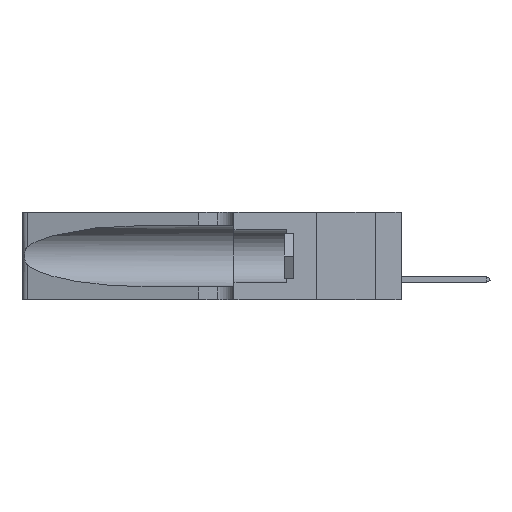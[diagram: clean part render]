
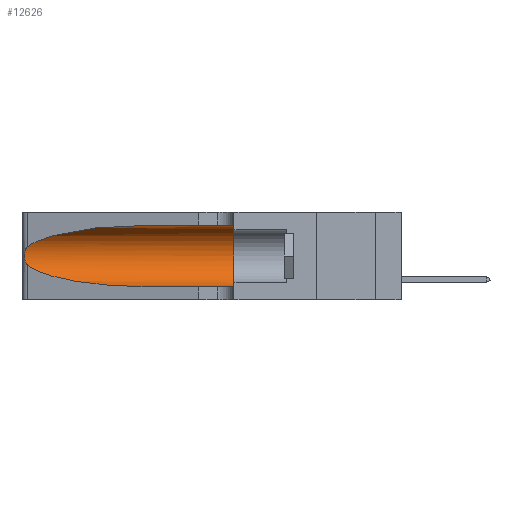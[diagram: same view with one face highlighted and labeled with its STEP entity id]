
A CAD part, left-side view. The second image highlights one B-rep face of the part: STEP entity #12626.
In plain terms, the highlighted cylindrical face has radius 3.308 mm (diameter 6.617 mm), a partial arc.
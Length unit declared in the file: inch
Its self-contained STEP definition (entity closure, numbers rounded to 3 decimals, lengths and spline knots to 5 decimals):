
#149 = DIRECTION ( 'NONE',  ( 0., 1., 0. ) ) ;
#244 = AXIS2_PLACEMENT_3D ( 'NONE', #2446, #10151, #14197 ) ;
#538 = CARTESIAN_POINT ( 'NONE',  ( 0.1305, 0.35, 0.05475 ) ) ;
#945 = CARTESIAN_POINT ( 'NONE',  ( 0.25487, 1.22718, 0.22369 ) ) ;
#1128 = EDGE_CURVE ( 'NONE', #13050, #4423, #2606, .T. ) ;
#2004 = ORIENTED_EDGE ( 'NONE', *, *, #10098, .T. ) ;
#2446 = CARTESIAN_POINT ( 'NONE',  ( 0.1305, 1.61858, 0.185 ) ) ;
#2606 = B_SPLINE_CURVE_WITH_KNOTS ( 'NONE', 3,
 ( #945, #4866, #18875, #8813, #20917, #10826, #5034, #8907, #22901, #22994, #10918, #24805, #25061, #9157 ),
 .UNSPECIFIED., .F., .F.,
 ( 4, 2, 2, 2, 2, 2, 4 ),
 ( 0., 0.00027, 0.00053, 0.00107, 0.0016, 0.00187, 0.00214 ),
 .UNSPECIFIED. ) ;
#3045 = FACE_OUTER_BOUND ( 'NONE', #23670, .T. ) ;
#3299 = DIRECTION ( 'NONE',  ( 0., -1., 0. ) ) ;
#4108 = CIRCLE ( 'NONE', #12021, 0.13025 ) ;
#4423 = VERTEX_POINT ( 'NONE', #16565 ) ;
#4842 = LINE ( 'NONE', #13563, #21802 ) ;
#4866 = CARTESIAN_POINT ( 'NONE',  ( 0.25555, 1.22994, 0.2215 ) ) ;
#5034 = CARTESIAN_POINT ( 'NONE',  ( 0.26075, 1.23896, 0.19203 ) ) ;
#5243 = CARTESIAN_POINT ( 'NONE',  ( 0.2373, 1.15595, 0.28018 ) ) ;
#6043 = VERTEX_POINT ( 'NONE', #14174 ) ;
#7356 = CARTESIAN_POINT ( 'NONE',  ( 0.18966, 0.96281, 0.31525 ) ) ;
#8057 =( BOUNDED_CURVE ( )  B_SPLINE_CURVE ( 3, ( #17282, #7356, #5243, #21306 ),
 .UNSPECIFIED., .F., .T. ) 
 B_SPLINE_CURVE_WITH_KNOTS ( ( 4, 4 ),
 ( 1.5708, 2.84003 ),
 .UNSPECIFIED. ) 
 CURVE ( )  GEOMETRIC_REPRESENTATION_ITEM ( )  RATIONAL_B_SPLINE_CURVE ( ( 1., 0.87, 0.87, 1. ) ) 
 REPRESENTATION_ITEM ( '' )  );
#8094 = VERTEX_POINT ( 'NONE', #538 ) ;
#8813 = CARTESIAN_POINT ( 'NONE',  ( 0.25787, 1.23484, 0.2124 ) ) ;
#8861 = CARTESIAN_POINT ( 'NONE',  ( 0.25487, 1.22718, 0.14631 ) ) ;
#8907 = CARTESIAN_POINT ( 'NONE',  ( 0.26075, 1.23896, 0.178 ) ) ;
#8988 = DIRECTION ( 'NONE',  ( 0., -1., 0. ) ) ;
#9157 = CARTESIAN_POINT ( 'NONE',  ( 0.25487, 1.22718, 0.14631 ) ) ;
#10098 = EDGE_CURVE ( 'NONE', #13844, #8094, #10925, .T. ) ;
#10126 = DIRECTION ( 'NONE',  ( 0., 0., 1. ) ) ;
#10151 = DIRECTION ( 'NONE',  ( 0., -1., 0. ) ) ;
#10527 = CARTESIAN_POINT ( 'NONE',  ( 0.2373, 1.15595, 0.08982 ) ) ;
#10826 = CARTESIAN_POINT ( 'NONE',  ( 0.26018, 1.23835, 0.19895 ) ) ;
#10918 = CARTESIAN_POINT ( 'NONE',  ( 0.25789, 1.23486, 0.15765 ) ) ;
#10925 = LINE ( 'NONE', #23768, #11554 ) ;
#11221 = CARTESIAN_POINT ( 'NONE',  ( 0.18966, 0.96281, 0.05475 ) ) ;
#11554 = VECTOR ( 'NONE', #8988, 39.37008 ) ;
#12021 = AXIS2_PLACEMENT_3D ( 'NONE', #12308, #149, #10126 ) ;
#12260 = CARTESIAN_POINT ( 'NONE',  ( 0.1305, 0.72297, 0.05475 ) ) ;
#12274 = CARTESIAN_POINT ( 'NONE',  ( 0.1305, 0.35, 0.31525 ) ) ;
#12308 = CARTESIAN_POINT ( 'NONE',  ( 0.1305, 0.35, 0.185 ) ) ;
#12352 = VERTEX_POINT ( 'NONE', #12274 ) ;
#12369 = EDGE_CURVE ( 'NONE', #4423, #13844, #13871, .T. ) ;
#12626 = ADVANCED_FACE ( 'NONE', ( #3045 ), #23665, .F. ) ;
#13050 = VERTEX_POINT ( 'NONE', #25778 ) ;
#13269 = CARTESIAN_POINT ( 'NONE',  ( 0.1305, 0.72297, 0.05475 ) ) ;
#13563 = CARTESIAN_POINT ( 'NONE',  ( 0.1305, 1.61858, 0.31525 ) ) ;
#13749 = ORIENTED_EDGE ( 'NONE', *, *, #1128, .T. ) ;
#13844 = VERTEX_POINT ( 'NONE', #12260 ) ;
#13871 =( BOUNDED_CURVE ( )  B_SPLINE_CURVE ( 3, ( #8861, #10527, #11221, #13269 ),
 .UNSPECIFIED., .F., .T. ) 
 B_SPLINE_CURVE_WITH_KNOTS ( ( 4, 4 ),
 ( 3.44316, 4.71239 ),
 .UNSPECIFIED. ) 
 CURVE ( )  GEOMETRIC_REPRESENTATION_ITEM ( )  RATIONAL_B_SPLINE_CURVE ( ( 1., 0.87, 0.87, 1. ) ) 
 REPRESENTATION_ITEM ( '' )  );
#14174 = CARTESIAN_POINT ( 'NONE',  ( 0.1305, 0.72297, 0.31525 ) ) ;
#14197 = DIRECTION ( 'NONE',  ( 0., 0., -1. ) ) ;
#14296 = ORIENTED_EDGE ( 'NONE', *, *, #15619, .F. ) ;
#15619 = EDGE_CURVE ( 'NONE', #12352, #8094, #4108, .T. ) ;
#16565 = CARTESIAN_POINT ( 'NONE',  ( 0.25487, 1.22718, 0.14631 ) ) ;
#16695 = ORIENTED_EDGE ( 'NONE', *, *, #21249, .F. ) ;
#17282 = CARTESIAN_POINT ( 'NONE',  ( 0.1305, 0.72297, 0.31525 ) ) ;
#18875 = CARTESIAN_POINT ( 'NONE',  ( 0.25639, 1.23184, 0.21858 ) ) ;
#18878 = ORIENTED_EDGE ( 'NONE', *, *, #12369, .T. ) ;
#20072 = EDGE_CURVE ( 'NONE', #6043, #13050, #8057, .T. ) ;
#20917 = CARTESIAN_POINT ( 'NONE',  ( 0.25854, 1.2359, 0.20912 ) ) ;
#21065 = ORIENTED_EDGE ( 'NONE', *, *, #20072, .T. ) ;
#21249 = EDGE_CURVE ( 'NONE', #6043, #12352, #4842, .T. ) ;
#21306 = CARTESIAN_POINT ( 'NONE',  ( 0.25487, 1.22718, 0.22369 ) ) ;
#21802 = VECTOR ( 'NONE', #3299, 39.37008 ) ;
#22901 = CARTESIAN_POINT ( 'NONE',  ( 0.26017, 1.23833, 0.17102 ) ) ;
#22994 = CARTESIAN_POINT ( 'NONE',  ( 0.25856, 1.23593, 0.16098 ) ) ;
#23665 = CYLINDRICAL_SURFACE ( 'NONE', #244, 0.13025 ) ;
#23670 = EDGE_LOOP ( 'NONE', ( #21065, #13749, #18878, #2004, #14296, #16695 ) ) ;
#23768 = CARTESIAN_POINT ( 'NONE',  ( 0.1305, 1.61858, 0.05475 ) ) ;
#24805 = CARTESIAN_POINT ( 'NONE',  ( 0.25639, 1.23186, 0.15144 ) ) ;
#25061 = CARTESIAN_POINT ( 'NONE',  ( 0.25555, 1.22993, 0.14849 ) ) ;
#25778 = CARTESIAN_POINT ( 'NONE',  ( 0.25487, 1.22718, 0.22369 ) ) ;
